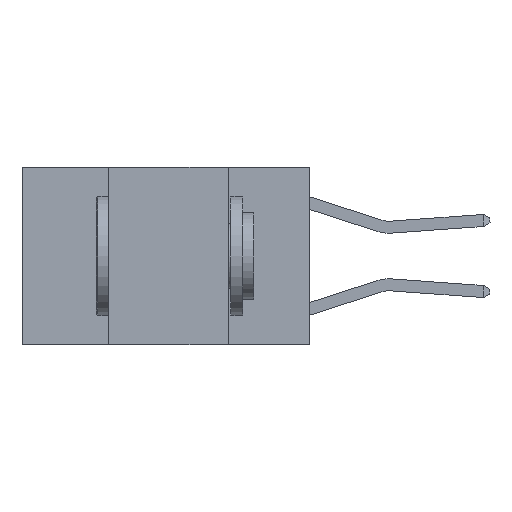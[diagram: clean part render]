
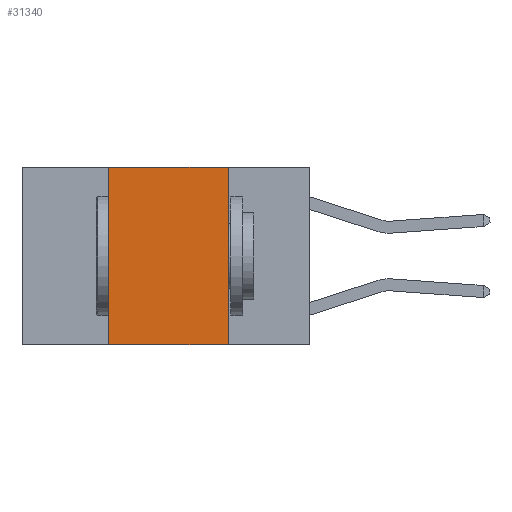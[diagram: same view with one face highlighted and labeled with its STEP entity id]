
A CAD part, left-side view. The second image highlights one B-rep face of the part: STEP entity #31340.
In plain terms, the highlighted planar face has unit normal (-1, 0, 0).
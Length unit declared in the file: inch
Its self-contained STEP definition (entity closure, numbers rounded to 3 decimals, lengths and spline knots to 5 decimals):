
#239 = VECTOR ( 'NONE', #26113, 39.37008 ) ;
#1852 = LINE ( 'NONE', #8565, #239 ) ;
#2115 = CARTESIAN_POINT ( 'NONE',  ( 0., 0.42, -0.37 ) ) ;
#2322 = ORIENTED_EDGE ( 'NONE', *, *, #16200, .F. ) ;
#3163 = LINE ( 'NONE', #6170, #9835 ) ;
#3315 = VERTEX_POINT ( 'NONE', #15009 ) ;
#5023 = VERTEX_POINT ( 'NONE', #20315 ) ;
#5230 = EDGE_CURVE ( 'NONE', #5023, #31860, #1852, .T. ) ;
#6170 = CARTESIAN_POINT ( 'NONE',  ( 0., 0.42, 0. ) ) ;
#6399 = DIRECTION ( 'NONE',  ( 1., 0., 0. ) ) ;
#7006 = EDGE_LOOP ( 'NONE', ( #14946, #21559, #2322, #16527 ) ) ;
#7748 = EDGE_CURVE ( 'NONE', #15326, #3315, #10012, .T. ) ;
#8565 = CARTESIAN_POINT ( 'NONE',  ( 0., 0.6, 0. ) ) ;
#8683 = DIRECTION ( 'NONE',  ( 0., 0., 1. ) ) ;
#9268 = FACE_OUTER_BOUND ( 'NONE', #7006, .T. ) ;
#9835 = VECTOR ( 'NONE', #8683, 39.37008 ) ;
#10012 = LINE ( 'NONE', #25281, #29225 ) ;
#14852 = CARTESIAN_POINT ( 'NONE',  ( 0., 0.17, 0. ) ) ;
#14946 = ORIENTED_EDGE ( 'NONE', *, *, #19519, .F. ) ;
#15009 = CARTESIAN_POINT ( 'NONE',  ( 0., 0.17, -0.37 ) ) ;
#15326 = VERTEX_POINT ( 'NONE', #2115 ) ;
#15713 = AXIS2_PLACEMENT_3D ( 'NONE', #16339, #6399, #23985 ) ;
#16200 = EDGE_CURVE ( 'NONE', #15326, #5023, #3163, .T. ) ;
#16339 = CARTESIAN_POINT ( 'NONE',  ( 0., 0.6, 0. ) ) ;
#16527 = ORIENTED_EDGE ( 'NONE', *, *, #7748, .T. ) ;
#16771 = DIRECTION ( 'NONE',  ( 0., 0., -1. ) ) ;
#18243 = VECTOR ( 'NONE', #16771, 39.37008 ) ;
#19519 = EDGE_CURVE ( 'NONE', #31860, #3315, #22537, .T. ) ;
#20315 = CARTESIAN_POINT ( 'NONE',  ( 0., 0.42, 0. ) ) ;
#21426 = PLANE ( 'NONE',  #15713 ) ;
#21559 = ORIENTED_EDGE ( 'NONE', *, *, #5230, .F. ) ;
#22537 = LINE ( 'NONE', #26707, #18243 ) ;
#23985 = DIRECTION ( 'NONE',  ( 0., 0., -1. ) ) ;
#25281 = CARTESIAN_POINT ( 'NONE',  ( 0., 0.6, -0.37 ) ) ;
#26113 = DIRECTION ( 'NONE',  ( 0., -1., 0. ) ) ;
#26707 = CARTESIAN_POINT ( 'NONE',  ( 0., 0.17, 0. ) ) ;
#27810 = DIRECTION ( 'NONE',  ( 0., -1., 0. ) ) ;
#29225 = VECTOR ( 'NONE', #27810, 39.37008 ) ;
#31340 = ADVANCED_FACE ( 'NONE', ( #9268 ), #21426, .F. ) ;
#31860 = VERTEX_POINT ( 'NONE', #14852 ) ;
